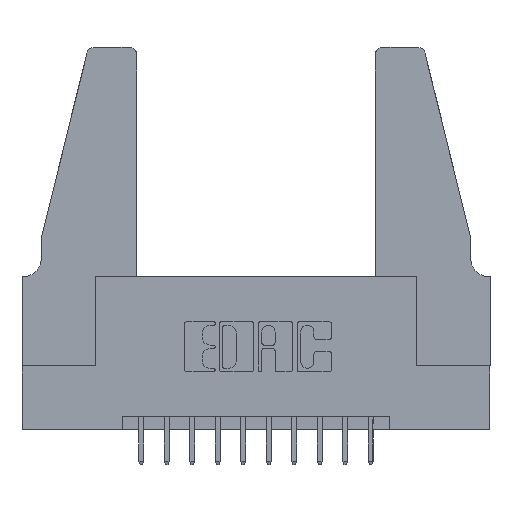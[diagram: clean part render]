
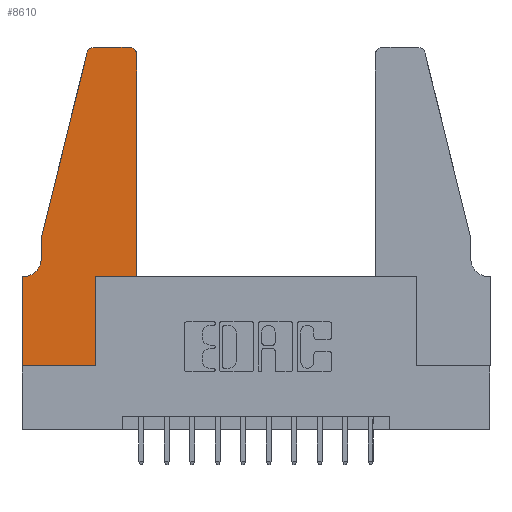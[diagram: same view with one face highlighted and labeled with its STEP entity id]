
A CAD part, top view. The second image highlights one B-rep face of the part: STEP entity #8610.
In plain terms, the highlighted planar face has unit normal (0, 0, 1).
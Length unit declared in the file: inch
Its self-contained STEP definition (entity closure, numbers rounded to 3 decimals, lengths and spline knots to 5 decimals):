
#44 = CARTESIAN_POINT ( 'NONE',  ( 0.0055, 0.35, 0.37 ) ) ;
#344 = ORIENTED_EDGE ( 'NONE', *, *, #961, .T. ) ;
#429 = VERTEX_POINT ( 'NONE', #12996 ) ;
#528 = VECTOR ( 'NONE', #3703, 39.37008 ) ;
#548 = EDGE_LOOP ( 'NONE', ( #5845, #13197, #14197, #4998, #7468, #5288, #344, #1594, #1207, #3792, #1888, #4662 ) ) ;
#575 = CARTESIAN_POINT ( 'NONE',  ( 0.284, 1.25, 0.37 ) ) ;
#707 = LINE ( 'NONE', #7265, #4702 ) ;
#721 = DIRECTION ( 'NONE',  ( 0., 0., 1. ) ) ;
#734 = EDGE_CURVE ( 'NONE', #2453, #5575, #2302, .T. ) ;
#961 = EDGE_CURVE ( 'NONE', #429, #6495, #5423, .T. ) ;
#1013 = LINE ( 'NONE', #12160, #11796 ) ;
#1154 = CARTESIAN_POINT ( 'NONE',  ( 0.25487, 1.22718, 0.37 ) ) ;
#1200 = LINE ( 'NONE', #12121, #6315 ) ;
#1207 = ORIENTED_EDGE ( 'NONE', *, *, #9599, .T. ) ;
#1230 = LINE ( 'NONE', #7913, #2124 ) ;
#1263 = EDGE_CURVE ( 'NONE', #2483, #4990, #12494, .T. ) ;
#1473 = CARTESIAN_POINT ( 'NONE',  ( 0.4505, 0.35, 0.37 ) ) ;
#1594 = ORIENTED_EDGE ( 'NONE', *, *, #3906, .T. ) ;
#1799 = FACE_OUTER_BOUND ( 'NONE', #548, .T. ) ;
#1888 = ORIENTED_EDGE ( 'NONE', *, *, #7863, .T. ) ;
#2067 = VECTOR ( 'NONE', #12407, 39.37008 ) ;
#2124 = VECTOR ( 'NONE', #2552, 39.37008 ) ;
#2302 = LINE ( 'NONE', #7954, #2067 ) ;
#2453 = VERTEX_POINT ( 'NONE', #1154 ) ;
#2483 = VERTEX_POINT ( 'NONE', #13353 ) ;
#2552 = DIRECTION ( 'NONE',  ( 0., -1., 0. ) ) ;
#2626 = EDGE_CURVE ( 'NONE', #12884, #7759, #707, .T. ) ;
#3235 = CARTESIAN_POINT ( 'NONE',  ( 0.284, 1.22, 0.37 ) ) ;
#3339 = DIRECTION ( 'NONE',  ( 1., 0., 0. ) ) ;
#3635 = AXIS2_PLACEMENT_3D ( 'NONE', #10771, #721, #13558 ) ;
#3703 = DIRECTION ( 'NONE',  ( 0., 1., 0. ) ) ;
#3792 = ORIENTED_EDGE ( 'NONE', *, *, #2626, .T. ) ;
#3906 = EDGE_CURVE ( 'NONE', #6495, #9746, #1200, .T. ) ;
#4041 = DIRECTION ( 'NONE',  ( 0., -1., 0. ) ) ;
#4074 = CARTESIAN_POINT ( 'NONE',  ( 0.0755, 0.5, 0.37 ) ) ;
#4203 = DIRECTION ( 'NONE',  ( 0., 0., -1. ) ) ;
#4539 = CIRCLE ( 'NONE', #6396, 0.03 ) ;
#4662 = ORIENTED_EDGE ( 'NONE', *, *, #5020, .T. ) ;
#4702 = VECTOR ( 'NONE', #9672, 39.37008 ) ;
#4990 = VERTEX_POINT ( 'NONE', #575 ) ;
#4998 = ORIENTED_EDGE ( 'NONE', *, *, #5230, .T. ) ;
#5020 = EDGE_CURVE ( 'NONE', #6194, #2483, #9385, .T. ) ;
#5230 = EDGE_CURVE ( 'NONE', #5575, #5287, #1230, .T. ) ;
#5287 = VERTEX_POINT ( 'NONE', #7844 ) ;
#5288 = ORIENTED_EDGE ( 'NONE', *, *, #14171, .T. ) ;
#5313 = DIRECTION ( 'NONE',  ( 0., 0., 1. ) ) ;
#5318 = AXIS2_PLACEMENT_3D ( 'NONE', #6307, #4203, #12999 ) ;
#5423 = LINE ( 'NONE', #6364, #8382 ) ;
#5539 = CIRCLE ( 'NONE', #5318, 0.07 ) ;
#5575 = VERTEX_POINT ( 'NONE', #4074 ) ;
#5589 = CARTESIAN_POINT ( 'NONE',  ( 0.2865, 0., 0.37 ) ) ;
#5646 = AXIS2_PLACEMENT_3D ( 'NONE', #11798, #6308, #7201 ) ;
#5686 = LINE ( 'NONE', #10488, #8052 ) ;
#5845 = ORIENTED_EDGE ( 'NONE', *, *, #1263, .T. ) ;
#6096 = DIRECTION ( 'NONE',  ( -1., 0., 0. ) ) ;
#6194 = VERTEX_POINT ( 'NONE', #9449 ) ;
#6307 = CARTESIAN_POINT ( 'NONE',  ( 0.0055, 0.42, 0.37 ) ) ;
#6308 = DIRECTION ( 'NONE',  ( 0., 0., 1. ) ) ;
#6315 = VECTOR ( 'NONE', #3339, 39.37008 ) ;
#6364 = CARTESIAN_POINT ( 'NONE',  ( 0., 0., 0.37 ) ) ;
#6396 = AXIS2_PLACEMENT_3D ( 'NONE', #3235, #5313, #9841 ) ;
#6495 = VERTEX_POINT ( 'NONE', #13704 ) ;
#6836 = VERTEX_POINT ( 'NONE', #44 ) ;
#7091 = DIRECTION ( 'NONE',  ( -1., 0., 0. ) ) ;
#7201 = DIRECTION ( 'NONE',  ( 1., 0., 0. ) ) ;
#7265 = CARTESIAN_POINT ( 'NONE',  ( 0.4505, 0.35, 0.37 ) ) ;
#7468 = ORIENTED_EDGE ( 'NONE', *, *, #13072, .T. ) ;
#7759 = VERTEX_POINT ( 'NONE', #1473 ) ;
#7844 = CARTESIAN_POINT ( 'NONE',  ( 0.0755, 0.42, 0.37 ) ) ;
#7863 = EDGE_CURVE ( 'NONE', #7759, #6194, #12381, .T. ) ;
#7913 = CARTESIAN_POINT ( 'NONE',  ( 0.0755, 0.5, 0.37 ) ) ;
#7954 = CARTESIAN_POINT ( 'NONE',  ( 0.0755, 0.5, 0.37 ) ) ;
#8005 = CARTESIAN_POINT ( 'NONE',  ( 0.2865, 0.35, 0.37 ) ) ;
#8052 = VECTOR ( 'NONE', #6096, 39.37008 ) ;
#8180 = CARTESIAN_POINT ( 'NONE',  ( 0.2605, 1.25, 0.37 ) ) ;
#8382 = VECTOR ( 'NONE', #4041, 39.37008 ) ;
#8610 = ADVANCED_FACE ( 'NONE', ( #1799 ), #10618, .T. ) ;
#9385 = CIRCLE ( 'NONE', #5646, 0.03 ) ;
#9449 = CARTESIAN_POINT ( 'NONE',  ( 0.4505, 1.22, 0.37 ) ) ;
#9563 = EDGE_CURVE ( 'NONE', #4990, #2453, #4539, .T. ) ;
#9599 = EDGE_CURVE ( 'NONE', #9746, #12884, #1013, .T. ) ;
#9672 = DIRECTION ( 'NONE',  ( 1., 0., 0. ) ) ;
#9746 = VERTEX_POINT ( 'NONE', #5589 ) ;
#9841 = DIRECTION ( 'NONE',  ( 1., 0., 0. ) ) ;
#10488 = CARTESIAN_POINT ( 'NONE',  ( 0.0755, 0.35, 0.37 ) ) ;
#10618 = PLANE ( 'NONE',  #3635 ) ;
#10771 = CARTESIAN_POINT ( 'NONE',  ( 0., 0.35, 0.37 ) ) ;
#10776 = DIRECTION ( 'NONE',  ( 0., 1., 0. ) ) ;
#11796 = VECTOR ( 'NONE', #10776, 39.37008 ) ;
#11798 = CARTESIAN_POINT ( 'NONE',  ( 0.4205, 1.22, 0.37 ) ) ;
#12121 = CARTESIAN_POINT ( 'NONE',  ( 0., 0., 0.37 ) ) ;
#12160 = CARTESIAN_POINT ( 'NONE',  ( 0.2865, 0.35, 0.37 ) ) ;
#12381 = LINE ( 'NONE', #13667, #528 ) ;
#12407 = DIRECTION ( 'NONE',  ( -0.239, -0.971, 0. ) ) ;
#12494 = LINE ( 'NONE', #8180, #13036 ) ;
#12884 = VERTEX_POINT ( 'NONE', #8005 ) ;
#12996 = CARTESIAN_POINT ( 'NONE',  ( 0., 0.35, 0.37 ) ) ;
#12999 = DIRECTION ( 'NONE',  ( -1., 0., 0. ) ) ;
#13036 = VECTOR ( 'NONE', #7091, 39.37008 ) ;
#13072 = EDGE_CURVE ( 'NONE', #5287, #6836, #5539, .T. ) ;
#13197 = ORIENTED_EDGE ( 'NONE', *, *, #9563, .T. ) ;
#13353 = CARTESIAN_POINT ( 'NONE',  ( 0.4205, 1.25, 0.37 ) ) ;
#13558 = DIRECTION ( 'NONE',  ( 1., 0., 0. ) ) ;
#13667 = CARTESIAN_POINT ( 'NONE',  ( 0.4505, 0.35, 0.37 ) ) ;
#13704 = CARTESIAN_POINT ( 'NONE',  ( 0., 0., 0.37 ) ) ;
#14171 = EDGE_CURVE ( 'NONE', #6836, #429, #5686, .T. ) ;
#14197 = ORIENTED_EDGE ( 'NONE', *, *, #734, .T. ) ;
